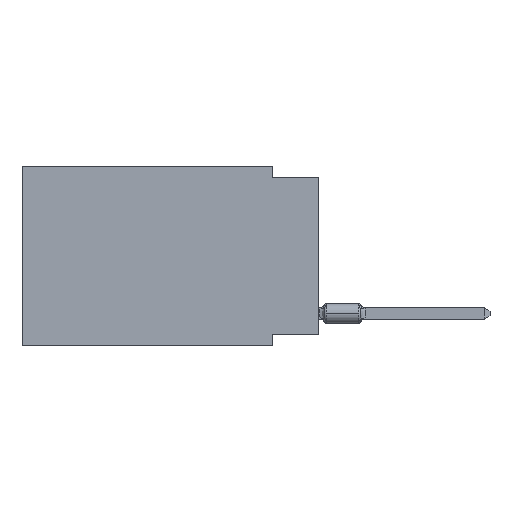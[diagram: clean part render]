
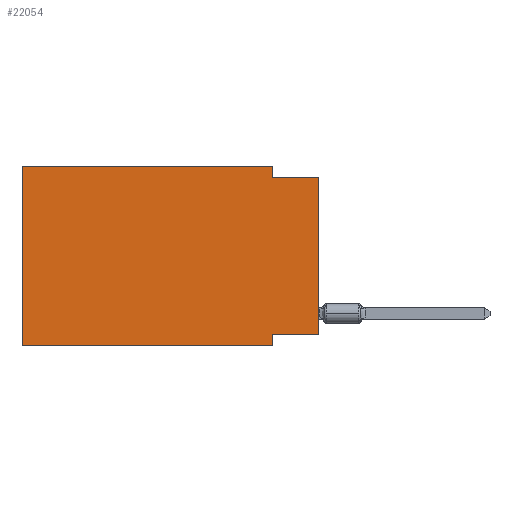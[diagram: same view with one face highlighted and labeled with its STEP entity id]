
A CAD part, left-side view. The second image highlights one B-rep face of the part: STEP entity #22054.
In plain terms, the highlighted planar face has unit normal (-1, 0, 0).
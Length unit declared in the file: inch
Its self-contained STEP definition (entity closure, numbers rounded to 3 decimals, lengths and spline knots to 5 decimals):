
#2036 = LINE ( 'NONE', #12224, #2967 ) ;
#2294 = VERTEX_POINT ( 'NONE', #14599 ) ;
#2834 = ORIENTED_EDGE ( 'NONE', *, *, #13146, .F. ) ;
#2967 = VECTOR ( 'NONE', #20923, 39.37008 ) ;
#5639 = VERTEX_POINT ( 'NONE', #8075 ) ;
#5689 = EDGE_CURVE ( 'NONE', #2294, #49469, #34465, .T. ) ;
#6066 = EDGE_CURVE ( 'NONE', #2294, #28854, #35595, .T. ) ;
#7447 = CARTESIAN_POINT ( 'NONE',  ( 0., 0., -0.025 ) ) ;
#8075 = CARTESIAN_POINT ( 'NONE',  ( 0., 0.645, -0.39 ) ) ;
#8600 = VECTOR ( 'NONE', #29520, 39.37008 ) ;
#9019 = LINE ( 'NONE', #27324, #28164 ) ;
#9138 = DIRECTION ( 'NONE',  ( 0., 0., -1. ) ) ;
#9962 = VECTOR ( 'NONE', #18010, 39.37008 ) ;
#11211 = EDGE_CURVE ( 'NONE', #51084, #26903, #30393, .T. ) ;
#11215 = CARTESIAN_POINT ( 'NONE',  ( 0., 0.1, 0. ) ) ;
#11714 = VECTOR ( 'NONE', #11757, 39.37008 ) ;
#11757 = DIRECTION ( 'NONE',  ( 0., -1., 0. ) ) ;
#12059 = CARTESIAN_POINT ( 'NONE',  ( 0., 0., -0.025 ) ) ;
#12224 = CARTESIAN_POINT ( 'NONE',  ( 0., 0.645, 0. ) ) ;
#12393 = ORIENTED_EDGE ( 'NONE', *, *, #6066, .T. ) ;
#13146 = EDGE_CURVE ( 'NONE', #23068, #51084, #2036, .T. ) ;
#14175 = FACE_OUTER_BOUND ( 'NONE', #29921, .T. ) ;
#14599 = CARTESIAN_POINT ( 'NONE',  ( 0., 0., -0.365 ) ) ;
#17999 = EDGE_CURVE ( 'NONE', #5639, #54538, #9019, .T. ) ;
#18010 = DIRECTION ( 'NONE',  ( 0., 0., 1. ) ) ;
#18999 = DIRECTION ( 'NONE',  ( 0., 0., -1. ) ) ;
#19274 = CARTESIAN_POINT ( 'NONE',  ( 0., 0.645, 0. ) ) ;
#20770 = CARTESIAN_POINT ( 'NONE',  ( 0., 0.1, -0.39 ) ) ;
#20923 = DIRECTION ( 'NONE',  ( 0., -1., 0. ) ) ;
#22054 = ADVANCED_FACE ( 'NONE', ( #14175 ), #40912, .F. ) ;
#23068 = VERTEX_POINT ( 'NONE', #57433 ) ;
#23075 = CARTESIAN_POINT ( 'NONE',  ( 0., 0.645, 0. ) ) ;
#23679 = AXIS2_PLACEMENT_3D ( 'NONE', #19274, #27393, #18999 ) ;
#26015 = DIRECTION ( 'NONE',  ( 0., 0., 1. ) ) ;
#26051 = ORIENTED_EDGE ( 'NONE', *, *, #5689, .F. ) ;
#26094 = ORIENTED_EDGE ( 'NONE', *, *, #58847, .F. ) ;
#26903 = VERTEX_POINT ( 'NONE', #52191 ) ;
#27324 = CARTESIAN_POINT ( 'NONE',  ( 0., 0.645, -0.39 ) ) ;
#27393 = DIRECTION ( 'NONE',  ( 1., 0., 0. ) ) ;
#28164 = VECTOR ( 'NONE', #45907, 39.37008 ) ;
#28854 = VERTEX_POINT ( 'NONE', #7447 ) ;
#29520 = DIRECTION ( 'NONE',  ( 0., 0., -1. ) ) ;
#29921 = EDGE_LOOP ( 'NONE', ( #12393, #52640, #39696, #2834, #42340, #56201, #26094, #26051 ) ) ;
#30393 = LINE ( 'NONE', #11215, #8600 ) ;
#32558 = CARTESIAN_POINT ( 'NONE',  ( 0., 0.1, -0.365 ) ) ;
#33287 = EDGE_CURVE ( 'NONE', #5639, #23068, #40504, .T. ) ;
#34465 = LINE ( 'NONE', #53086, #57057 ) ;
#34847 = LINE ( 'NONE', #12059, #11714 ) ;
#35595 = LINE ( 'NONE', #39831, #49415 ) ;
#39696 = ORIENTED_EDGE ( 'NONE', *, *, #11211, .F. ) ;
#39699 = VECTOR ( 'NONE', #9138, 39.37008 ) ;
#39831 = CARTESIAN_POINT ( 'NONE',  ( 0., 0., 0. ) ) ;
#40504 = LINE ( 'NONE', #23075, #9962 ) ;
#40900 = EDGE_CURVE ( 'NONE', #26903, #28854, #34847, .T. ) ;
#40912 = PLANE ( 'NONE',  #23679 ) ;
#41830 = LINE ( 'NONE', #50549, #39699 ) ;
#42340 = ORIENTED_EDGE ( 'NONE', *, *, #33287, .F. ) ;
#45907 = DIRECTION ( 'NONE',  ( 0., -1., 0. ) ) ;
#47493 = CARTESIAN_POINT ( 'NONE',  ( 0., 0.1, 0. ) ) ;
#49415 = VECTOR ( 'NONE', #26015, 39.37008 ) ;
#49469 = VERTEX_POINT ( 'NONE', #32558 ) ;
#50549 = CARTESIAN_POINT ( 'NONE',  ( 0., 0.1, -0.39 ) ) ;
#51084 = VERTEX_POINT ( 'NONE', #47493 ) ;
#52191 = CARTESIAN_POINT ( 'NONE',  ( 0., 0.1, -0.025 ) ) ;
#52640 = ORIENTED_EDGE ( 'NONE', *, *, #40900, .F. ) ;
#53086 = CARTESIAN_POINT ( 'NONE',  ( 0., 0., -0.365 ) ) ;
#54538 = VERTEX_POINT ( 'NONE', #20770 ) ;
#56201 = ORIENTED_EDGE ( 'NONE', *, *, #17999, .T. ) ;
#57057 = VECTOR ( 'NONE', #57321, 39.37008 ) ;
#57321 = DIRECTION ( 'NONE',  ( 0., 1., 0. ) ) ;
#57433 = CARTESIAN_POINT ( 'NONE',  ( 0., 0.645, 0. ) ) ;
#58847 = EDGE_CURVE ( 'NONE', #49469, #54538, #41830, .T. ) ;
